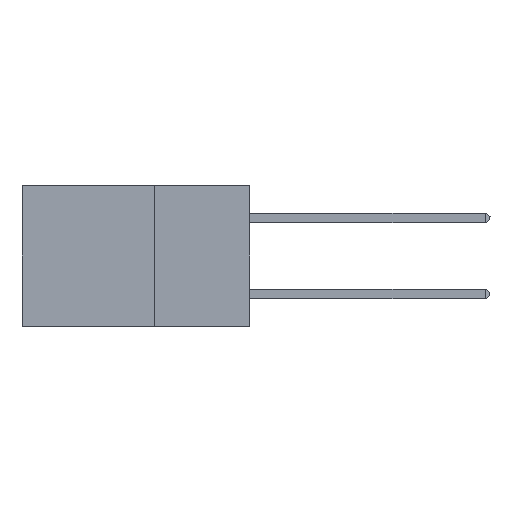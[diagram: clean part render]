
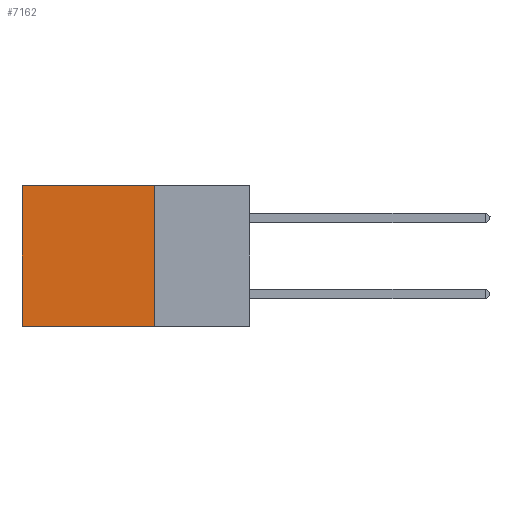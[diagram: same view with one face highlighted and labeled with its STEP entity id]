
A CAD part, left-side view. The second image highlights one B-rep face of the part: STEP entity #7162.
In plain terms, the highlighted planar face has unit normal (-1, 0, 0).
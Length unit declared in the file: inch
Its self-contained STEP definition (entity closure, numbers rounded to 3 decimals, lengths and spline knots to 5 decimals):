
#879 = VECTOR ( 'NONE', #2372, 39.37008 ) ;
#1104 = AXIS2_PLACEMENT_3D ( 'NONE', #14421, #8771, #2799 ) ;
#1163 = PLANE ( 'NONE',  #1104 ) ;
#1206 = VECTOR ( 'NONE', #18246, 39.37008 ) ;
#1399 = VECTOR ( 'NONE', #5829, 39.37008 ) ;
#1802 = EDGE_LOOP ( 'NONE', ( #18841, #6834, #12789, #3816 ) ) ;
#2171 = CARTESIAN_POINT ( 'NONE',  ( 0.2875, 0.6, 0. ) ) ;
#2372 = DIRECTION ( 'NONE',  ( 0., 0., -1. ) ) ;
#2678 = EDGE_CURVE ( 'NONE', #15586, #6302, #9532, .T. ) ;
#2799 = DIRECTION ( 'NONE',  ( 0., 0., -1. ) ) ;
#3121 = EDGE_CURVE ( 'NONE', #6302, #5161, #18229, .T. ) ;
#3262 = VERTEX_POINT ( 'NONE', #11369 ) ;
#3301 = CARTESIAN_POINT ( 'NONE',  ( 0.2875, 0.25, 0. ) ) ;
#3816 = ORIENTED_EDGE ( 'NONE', *, *, #6932, .T. ) ;
#5042 = CARTESIAN_POINT ( 'NONE',  ( 0.2875, 0.25, 0. ) ) ;
#5161 = VERTEX_POINT ( 'NONE', #13554 ) ;
#5829 = DIRECTION ( 'NONE',  ( 0., 1., 0. ) ) ;
#6302 = VERTEX_POINT ( 'NONE', #7160 ) ;
#6630 = CARTESIAN_POINT ( 'NONE',  ( 0.2875, 0.25, 0. ) ) ;
#6834 = ORIENTED_EDGE ( 'NONE', *, *, #3121, .F. ) ;
#6932 = EDGE_CURVE ( 'NONE', #15586, #3262, #16756, .T. ) ;
#7160 = CARTESIAN_POINT ( 'NONE',  ( 0.2875, 0.25, -0.37 ) ) ;
#7162 = ADVANCED_FACE ( 'NONE', ( #17423 ), #1163, .F. ) ;
#8771 = DIRECTION ( 'NONE',  ( 1., 0., 0. ) ) ;
#9521 = LINE ( 'NONE', #2171, #1206 ) ;
#9532 = LINE ( 'NONE', #6630, #879 ) ;
#10899 = DIRECTION ( 'NONE',  ( 0., 1., 0. ) ) ;
#11369 = CARTESIAN_POINT ( 'NONE',  ( 0.2875, 0.6, 0. ) ) ;
#12586 = EDGE_CURVE ( 'NONE', #3262, #5161, #9521, .T. ) ;
#12789 = ORIENTED_EDGE ( 'NONE', *, *, #2678, .F. ) ;
#13554 = CARTESIAN_POINT ( 'NONE',  ( 0.2875, 0.6, -0.37 ) ) ;
#13996 = CARTESIAN_POINT ( 'NONE',  ( 0.2875, 0.25, -0.37 ) ) ;
#14421 = CARTESIAN_POINT ( 'NONE',  ( 0.2875, 0.25, 0. ) ) ;
#14920 = VECTOR ( 'NONE', #10899, 39.37008 ) ;
#15586 = VERTEX_POINT ( 'NONE', #5042 ) ;
#16756 = LINE ( 'NONE', #3301, #1399 ) ;
#17423 = FACE_OUTER_BOUND ( 'NONE', #1802, .T. ) ;
#18229 = LINE ( 'NONE', #13996, #14920 ) ;
#18246 = DIRECTION ( 'NONE',  ( 0., 0., -1. ) ) ;
#18841 = ORIENTED_EDGE ( 'NONE', *, *, #12586, .T. ) ;
